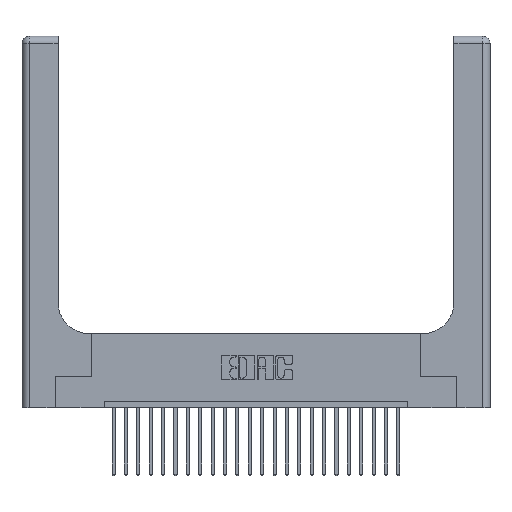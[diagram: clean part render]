
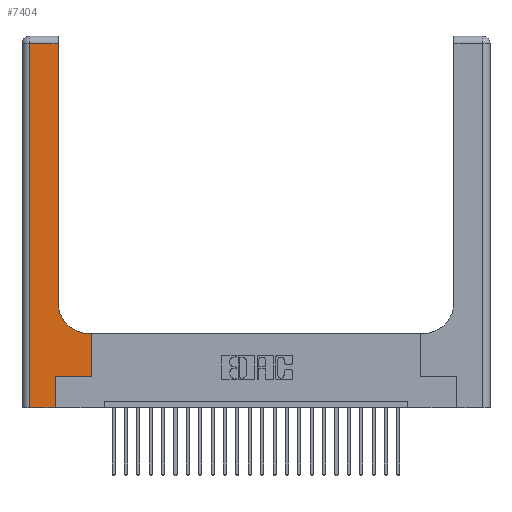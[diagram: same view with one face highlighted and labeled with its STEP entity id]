
A CAD part, top view. The second image highlights one B-rep face of the part: STEP entity #7404.
In plain terms, the highlighted planar face has unit normal (0, 0, 1).
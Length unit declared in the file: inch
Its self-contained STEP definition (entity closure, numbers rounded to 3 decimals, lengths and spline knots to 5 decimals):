
#534 = LINE ( 'NONE', #18682, #1162 ) ;
#1162 = VECTOR ( 'NONE', #10789, 39.37008 ) ;
#1781 = DIRECTION ( 'NONE',  ( 0., 1., 0. ) ) ;
#1936 = ORIENTED_EDGE ( 'NONE', *, *, #17089, .T. ) ;
#2023 = CARTESIAN_POINT ( 'NONE',  ( 0., 3., 0.37 ) ) ;
#2026 = EDGE_CURVE ( 'NONE', #18823, #24452, #4696, .T. ) ;
#3079 = EDGE_LOOP ( 'NONE', ( #3484, #5022, #24138, #22330, #16806, #7142, #4638, #1936, #8984 ) ) ;
#3199 = VERTEX_POINT ( 'NONE', #20651 ) ;
#3463 = VERTEX_POINT ( 'NONE', #21574 ) ;
#3484 = ORIENTED_EDGE ( 'NONE', *, *, #8336, .T. ) ;
#4184 = VECTOR ( 'NONE', #9374, 39.37008 ) ;
#4267 = LINE ( 'NONE', #18296, #24100 ) ;
#4312 = DIRECTION ( 'NONE',  ( -1., 0., 0. ) ) ;
#4556 = DIRECTION ( 'NONE',  ( 1., 0., 0. ) ) ;
#4638 = ORIENTED_EDGE ( 'NONE', *, *, #8378, .T. ) ;
#4696 = CIRCLE ( 'NONE', #14196, 0.25 ) ;
#5022 = ORIENTED_EDGE ( 'NONE', *, *, #12639, .T. ) ;
#5542 = LINE ( 'NONE', #10526, #24166 ) ;
#6042 = CARTESIAN_POINT ( 'NONE',  ( 0.06, 0., 0.37 ) ) ;
#6053 = DIRECTION ( 'NONE',  ( 0., 1., 0. ) ) ;
#6301 = CARTESIAN_POINT ( 'NONE',  ( 0.5415, 0.85, 0.37 ) ) ;
#6312 = PLANE ( 'NONE',  #23616 ) ;
#6778 = VERTEX_POINT ( 'NONE', #8137 ) ;
#7142 = ORIENTED_EDGE ( 'NONE', *, *, #18252, .T. ) ;
#7314 = CARTESIAN_POINT ( 'NONE',  ( 0., 2.94, 0.37 ) ) ;
#7384 = EDGE_CURVE ( 'NONE', #7940, #6778, #24094, .T. ) ;
#7404 = ADVANCED_FACE ( 'NONE', ( #8264 ), #6312, .F. ) ;
#7732 = CARTESIAN_POINT ( 'NONE',  ( 0.2915, 2.94, 0.37 ) ) ;
#7940 = VERTEX_POINT ( 'NONE', #6042 ) ;
#8137 = CARTESIAN_POINT ( 'NONE',  ( 0.269, 0., 0.37 ) ) ;
#8264 = FACE_OUTER_BOUND ( 'NONE', #3079, .T. ) ;
#8336 = EDGE_CURVE ( 'NONE', #24452, #8373, #21545, .T. ) ;
#8373 = VERTEX_POINT ( 'NONE', #7732 ) ;
#8378 = EDGE_CURVE ( 'NONE', #15519, #3199, #14040, .T. ) ;
#8832 = DIRECTION ( 'NONE',  ( 0., 0., -1. ) ) ;
#8984 = ORIENTED_EDGE ( 'NONE', *, *, #2026, .T. ) ;
#9300 = DIRECTION ( 'NONE',  ( -1., 0., 0. ) ) ;
#9374 = DIRECTION ( 'NONE',  ( 0., 1., 0. ) ) ;
#10526 = CARTESIAN_POINT ( 'NONE',  ( 0.2915, 0.6, 0.37 ) ) ;
#10789 = DIRECTION ( 'NONE',  ( 1., 0., 0. ) ) ;
#12271 = DIRECTION ( 'NONE',  ( 0., 0., -1. ) ) ;
#12394 = CARTESIAN_POINT ( 'NONE',  ( 0.5585, 0.25, 0.37 ) ) ;
#12568 = DIRECTION ( 'NONE',  ( 0., -1., 0. ) ) ;
#12639 = EDGE_CURVE ( 'NONE', #8373, #3463, #22809, .T. ) ;
#12862 = VECTOR ( 'NONE', #9300, 39.37008 ) ;
#13687 = CARTESIAN_POINT ( 'NONE',  ( 0., 0., 0.37 ) ) ;
#14040 = LINE ( 'NONE', #25530, #4184 ) ;
#14196 = AXIS2_PLACEMENT_3D ( 'NONE', #6301, #12271, #20269 ) ;
#14842 = VECTOR ( 'NONE', #6053, 39.37008 ) ;
#15519 = VERTEX_POINT ( 'NONE', #12394 ) ;
#15814 = CARTESIAN_POINT ( 'NONE',  ( 0.269, 0., 0.37 ) ) ;
#16293 = VECTOR ( 'NONE', #4556, 39.37008 ) ;
#16806 = ORIENTED_EDGE ( 'NONE', *, *, #17216, .T. ) ;
#17089 = EDGE_CURVE ( 'NONE', #3199, #18823, #5542, .T. ) ;
#17216 = EDGE_CURVE ( 'NONE', #6778, #21955, #21367, .T. ) ;
#18150 = DIRECTION ( 'NONE',  ( -1., 0., 0. ) ) ;
#18252 = EDGE_CURVE ( 'NONE', #21955, #15519, #534, .T. ) ;
#18296 = CARTESIAN_POINT ( 'NONE',  ( 0.06, 3., 0.37 ) ) ;
#18682 = CARTESIAN_POINT ( 'NONE',  ( 0.269, 0.25, 0.37 ) ) ;
#18823 = VERTEX_POINT ( 'NONE', #23253 ) ;
#20269 = DIRECTION ( 'NONE',  ( 1., 0., 0. ) ) ;
#20649 = CARTESIAN_POINT ( 'NONE',  ( 0.269, 0.25, 0.37 ) ) ;
#20651 = CARTESIAN_POINT ( 'NONE',  ( 0.5585, 0.6, 0.37 ) ) ;
#21367 = LINE ( 'NONE', #15814, #14842 ) ;
#21545 = LINE ( 'NONE', #25271, #22799 ) ;
#21574 = CARTESIAN_POINT ( 'NONE',  ( 0.06, 2.94, 0.37 ) ) ;
#21955 = VERTEX_POINT ( 'NONE', #20649 ) ;
#22330 = ORIENTED_EDGE ( 'NONE', *, *, #7384, .T. ) ;
#22799 = VECTOR ( 'NONE', #1781, 39.37008 ) ;
#22809 = LINE ( 'NONE', #7314, #12862 ) ;
#23253 = CARTESIAN_POINT ( 'NONE',  ( 0.5415, 0.6, 0.37 ) ) ;
#23616 = AXIS2_PLACEMENT_3D ( 'NONE', #2023, #8832, #18150 ) ;
#24094 = LINE ( 'NONE', #13687, #16293 ) ;
#24100 = VECTOR ( 'NONE', #12568, 39.37008 ) ;
#24138 = ORIENTED_EDGE ( 'NONE', *, *, #25548, .T. ) ;
#24166 = VECTOR ( 'NONE', #4312, 39.37008 ) ;
#24452 = VERTEX_POINT ( 'NONE', #24965 ) ;
#24965 = CARTESIAN_POINT ( 'NONE',  ( 0.2915, 0.85, 0.37 ) ) ;
#25271 = CARTESIAN_POINT ( 'NONE',  ( 0.2915, 3., 0.37 ) ) ;
#25530 = CARTESIAN_POINT ( 'NONE',  ( 0.5585, 0.25, 0.37 ) ) ;
#25548 = EDGE_CURVE ( 'NONE', #3463, #7940, #4267, .T. ) ;
